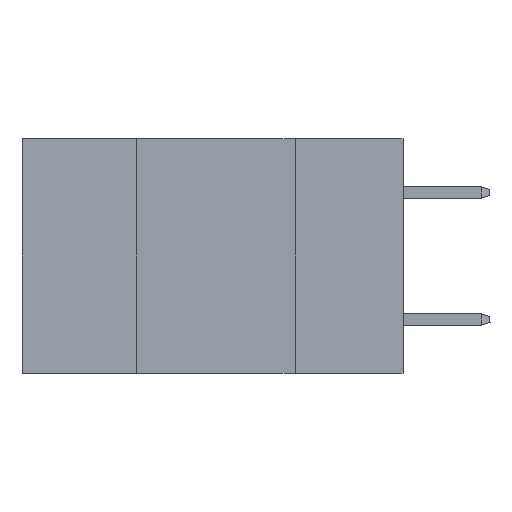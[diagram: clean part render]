
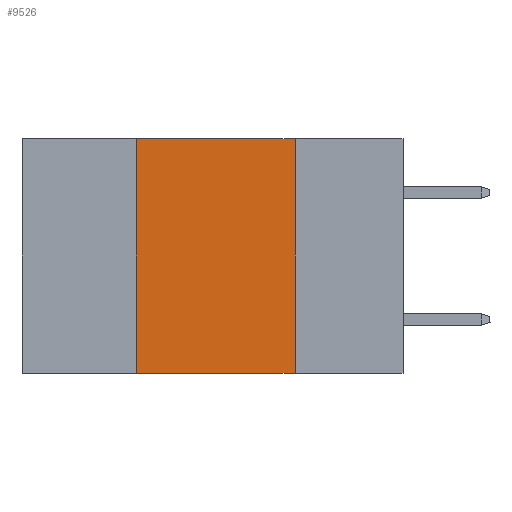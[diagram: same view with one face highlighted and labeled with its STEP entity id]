
A CAD part, left-side view. The second image highlights one B-rep face of the part: STEP entity #9526.
In plain terms, the highlighted planar face has unit normal (-1, 0, 0).
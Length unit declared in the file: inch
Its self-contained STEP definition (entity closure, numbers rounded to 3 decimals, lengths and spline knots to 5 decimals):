
#136 = CARTESIAN_POINT ( 'NONE',  ( 0., 0.42, -0.37 ) ) ;
#658 = EDGE_CURVE ( 'NONE', #11352, #4928, #2154, .T. ) ;
#828 = CARTESIAN_POINT ( 'NONE',  ( 0., 0.6, 0. ) ) ;
#1802 = VECTOR ( 'NONE', #1845, 39.37008 ) ;
#1845 = DIRECTION ( 'NONE',  ( 0., -1., 0. ) ) ;
#1877 = VECTOR ( 'NONE', #10728, 39.37008 ) ;
#2061 = VERTEX_POINT ( 'NONE', #10182 ) ;
#2154 = LINE ( 'NONE', #828, #1802 ) ;
#2500 = CARTESIAN_POINT ( 'NONE',  ( 0., 0.6, 0. ) ) ;
#3905 = FACE_OUTER_BOUND ( 'NONE', #9697, .T. ) ;
#3950 = AXIS2_PLACEMENT_3D ( 'NONE', #2500, #12280, #11020 ) ;
#4064 = VERTEX_POINT ( 'NONE', #136 ) ;
#4867 = DIRECTION ( 'NONE',  ( 0., -1., 0. ) ) ;
#4928 = VERTEX_POINT ( 'NONE', #9532 ) ;
#5663 = DIRECTION ( 'NONE',  ( 0., 0., 1. ) ) ;
#5739 = EDGE_CURVE ( 'NONE', #4064, #2061, #11979, .T. ) ;
#5828 = CARTESIAN_POINT ( 'NONE',  ( 0., 0.6, -0.37 ) ) ;
#6765 = LINE ( 'NONE', #11594, #15254 ) ;
#7139 = LINE ( 'NONE', #11895, #1877 ) ;
#7519 = PLANE ( 'NONE',  #3950 ) ;
#7911 = VECTOR ( 'NONE', #4867, 39.37008 ) ;
#9342 = CARTESIAN_POINT ( 'NONE',  ( 0., 0.42, 0. ) ) ;
#9526 = ADVANCED_FACE ( 'NONE', ( #3905 ), #7519, .F. ) ;
#9532 = CARTESIAN_POINT ( 'NONE',  ( 0., 0.17, 0. ) ) ;
#9697 = EDGE_LOOP ( 'NONE', ( #12408, #13752, #15224, #13096 ) ) ;
#10182 = CARTESIAN_POINT ( 'NONE',  ( 0., 0.17, -0.37 ) ) ;
#10290 = EDGE_CURVE ( 'NONE', #4064, #11352, #6765, .T. ) ;
#10728 = DIRECTION ( 'NONE',  ( 0., 0., -1. ) ) ;
#11020 = DIRECTION ( 'NONE',  ( 0., 0., -1. ) ) ;
#11352 = VERTEX_POINT ( 'NONE', #9342 ) ;
#11594 = CARTESIAN_POINT ( 'NONE',  ( 0., 0.42, 0. ) ) ;
#11895 = CARTESIAN_POINT ( 'NONE',  ( 0., 0.17, 0. ) ) ;
#11949 = EDGE_CURVE ( 'NONE', #4928, #2061, #7139, .T. ) ;
#11979 = LINE ( 'NONE', #5828, #7911 ) ;
#12280 = DIRECTION ( 'NONE',  ( 1., 0., 0. ) ) ;
#12408 = ORIENTED_EDGE ( 'NONE', *, *, #11949, .F. ) ;
#13096 = ORIENTED_EDGE ( 'NONE', *, *, #5739, .T. ) ;
#13752 = ORIENTED_EDGE ( 'NONE', *, *, #658, .F. ) ;
#15224 = ORIENTED_EDGE ( 'NONE', *, *, #10290, .F. ) ;
#15254 = VECTOR ( 'NONE', #5663, 39.37008 ) ;
